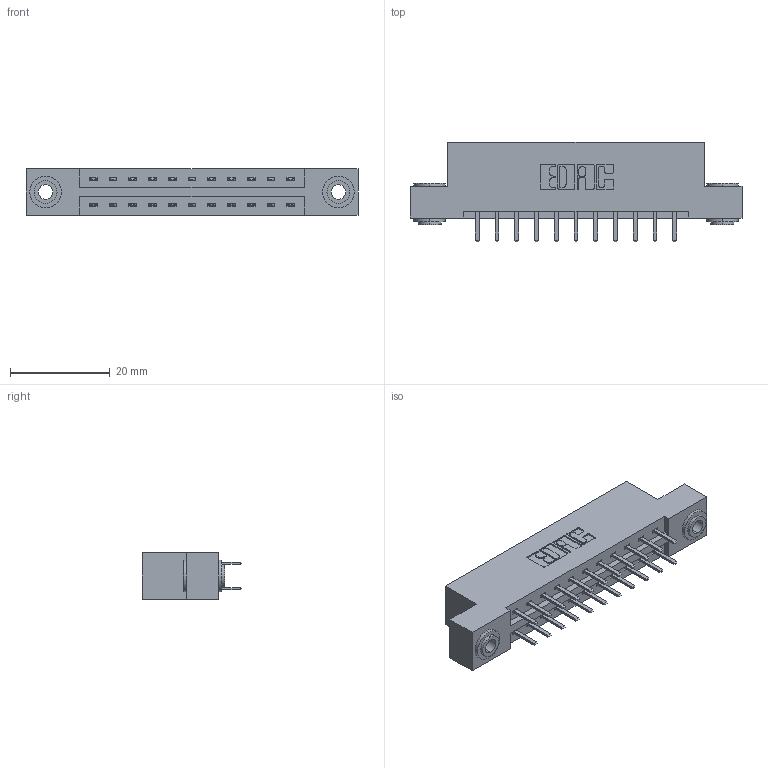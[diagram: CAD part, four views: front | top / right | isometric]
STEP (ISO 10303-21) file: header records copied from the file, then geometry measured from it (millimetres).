
FILE_DESCRIPTION (( 'STEP AP203' ), '1' );
FILE_NAME ('337-022-520-203.STEP', '2019-10-08T14:30:42', ( '' ), ( '' ), 'SwSTEP 2.0', 'SolidWorks 2016', '' );
FILE_SCHEMA (( 'CONFIG_CONTROL_DESIGN' ));
Length unit declared in the file: inch
Products named in the file (4): 337-022-520-203; 345-292-001_345-293-120; 345-250-002_345-250-002-102; 337 Part_Flush Mounting Lugs - 0.156 Dia-TH
Assembly tree (25 placements, depth 2):
  337-022-520-203
    337 Part_Flush Mounting Lugs - 0.156 Dia-TH
    345-292-001_345-293-120  x22
    345-250-002_345-250-002-102  x2
Bounding box: 66.6 x 20.02 x 9.4 mm (x, y, z)
Volume: 6615.8 mm3; surface area: 7374.9 mm2
Topology: 25 solids, 25 shells, 1428 faces, 4105 edges, 2674 vertices
Faces by surface type: plane 960, cylinder 460, cone 8
Entity records: 13302 total; most frequent: CARTESIAN_POINT 2253, ORIENTED_EDGE 2170, DIRECTION 1995, EDGE_CURVE 1085, VECTOR 929, LINE 929, VERTEX_POINT 718, AXIS2_PLACEMENT_3D 533
